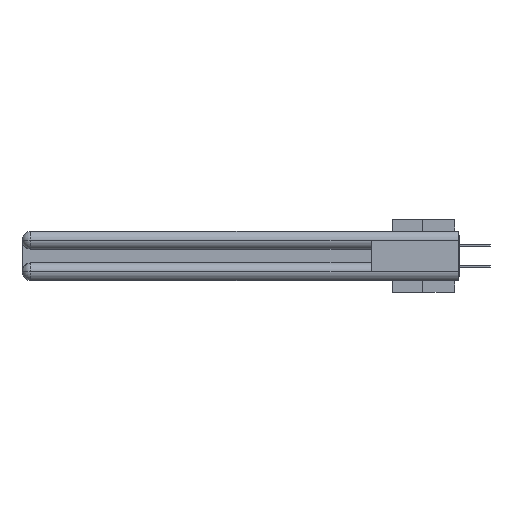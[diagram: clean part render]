
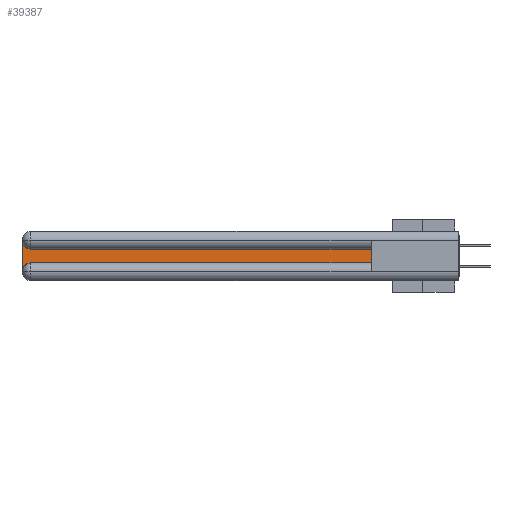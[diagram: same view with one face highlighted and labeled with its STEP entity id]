
A CAD part, left-side view. The second image highlights one B-rep face of the part: STEP entity #39387.
In plain terms, the highlighted planar face has unit normal (-1, 0, 0).
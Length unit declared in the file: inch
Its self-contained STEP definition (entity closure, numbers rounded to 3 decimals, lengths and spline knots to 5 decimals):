
#1821 = LINE ( 'NONE', #38456, #41019 ) ;
#2077 = VERTEX_POINT ( 'NONE', #18280 ) ;
#2661 = VECTOR ( 'NONE', #31508, 39.37008 ) ;
#4078 = LINE ( 'NONE', #7521, #40388 ) ;
#5227 = AXIS2_PLACEMENT_3D ( 'NONE', #21280, #36305, #42930 ) ;
#5736 = CIRCLE ( 'NONE', #5227, 0.06 ) ;
#5887 = CARTESIAN_POINT ( 'NONE',  ( 0.075, 3., -0.2775 ) ) ;
#7521 = CARTESIAN_POINT ( 'NONE',  ( 0.075, 0.6, -0.1225 ) ) ;
#7778 = LINE ( 'NONE', #32529, #10006 ) ;
#8079 = ORIENTED_EDGE ( 'NONE', *, *, #13243, .T. ) ;
#8795 = AXIS2_PLACEMENT_3D ( 'NONE', #41624, #34814, #13100 ) ;
#9459 = PLANE ( 'NONE',  #8795 ) ;
#10006 = VECTOR ( 'NONE', #14460, 39.37008 ) ;
#10050 = VERTEX_POINT ( 'NONE', #34421 ) ;
#11259 = LINE ( 'NONE', #41633, #2661 ) ;
#11621 = CARTESIAN_POINT ( 'NONE',  ( 0.075, 2.94, -0.2175 ) ) ;
#12959 = DIRECTION ( 'NONE',  ( 0., 0., -1. ) ) ;
#13100 = DIRECTION ( 'NONE',  ( 0., 0., -1. ) ) ;
#13243 = EDGE_CURVE ( 'NONE', #30678, #10050, #11259, .T. ) ;
#13375 = FACE_OUTER_BOUND ( 'NONE', #41332, .T. ) ;
#14460 = DIRECTION ( 'NONE',  ( 0., 0., 1. ) ) ;
#14841 = VERTEX_POINT ( 'NONE', #17853 ) ;
#16288 = AXIS2_PLACEMENT_3D ( 'NONE', #17641, #42916, #21264 ) ;
#17641 = CARTESIAN_POINT ( 'NONE',  ( 0.075, 2.94, -0.2775 ) ) ;
#17853 = CARTESIAN_POINT ( 'NONE',  ( 0.075, 2.94, -0.1225 ) ) ;
#18280 = CARTESIAN_POINT ( 'NONE',  ( 0.075, 0.6, -0.1225 ) ) ;
#18743 = CIRCLE ( 'NONE', #16288, 0.06 ) ;
#20013 = ORIENTED_EDGE ( 'NONE', *, *, #34995, .T. ) ;
#21264 = DIRECTION ( 'NONE',  ( 0., 0., -1. ) ) ;
#21280 = CARTESIAN_POINT ( 'NONE',  ( 0.075, 2.94, -0.0625 ) ) ;
#22581 = ORIENTED_EDGE ( 'NONE', *, *, #24065, .T. ) ;
#23924 = VERTEX_POINT ( 'NONE', #5887 ) ;
#24065 = EDGE_CURVE ( 'NONE', #10050, #2077, #7778, .T. ) ;
#24302 = CARTESIAN_POINT ( 'NONE',  ( 0.075, 3., -0.0625 ) ) ;
#25035 = ORIENTED_EDGE ( 'NONE', *, *, #44098, .T. ) ;
#25406 = VERTEX_POINT ( 'NONE', #24302 ) ;
#30678 = VERTEX_POINT ( 'NONE', #11621 ) ;
#31508 = DIRECTION ( 'NONE',  ( 0., -1., 0. ) ) ;
#32529 = CARTESIAN_POINT ( 'NONE',  ( 0.075, 0.6, -0.2175 ) ) ;
#33034 = DIRECTION ( 'NONE',  ( 0., 1., 0. ) ) ;
#34421 = CARTESIAN_POINT ( 'NONE',  ( 0.075, 0.6, -0.2175 ) ) ;
#34814 = DIRECTION ( 'NONE',  ( 1., 0., 0. ) ) ;
#34995 = EDGE_CURVE ( 'NONE', #25406, #23924, #1821, .T. ) ;
#36305 = DIRECTION ( 'NONE',  ( 1., 0., 0. ) ) ;
#38456 = CARTESIAN_POINT ( 'NONE',  ( 0.075, 3., -0.2175 ) ) ;
#39387 = ADVANCED_FACE ( 'NONE', ( #13375 ), #9459, .F. ) ;
#40388 = VECTOR ( 'NONE', #33034, 39.37008 ) ;
#40909 = ORIENTED_EDGE ( 'NONE', *, *, #41760, .T. ) ;
#41019 = VECTOR ( 'NONE', #12959, 39.37008 ) ;
#41332 = EDGE_LOOP ( 'NONE', ( #40909, #41495, #20013, #25035, #8079, #22581 ) ) ;
#41495 = ORIENTED_EDGE ( 'NONE', *, *, #42522, .T. ) ;
#41624 = CARTESIAN_POINT ( 'NONE',  ( 0.075, 3., -0.1225 ) ) ;
#41633 = CARTESIAN_POINT ( 'NONE',  ( 0.075, 0.6, -0.2175 ) ) ;
#41760 = EDGE_CURVE ( 'NONE', #2077, #14841, #4078, .T. ) ;
#42522 = EDGE_CURVE ( 'NONE', #14841, #25406, #5736, .T. ) ;
#42916 = DIRECTION ( 'NONE',  ( 1., 0., 0. ) ) ;
#42930 = DIRECTION ( 'NONE',  ( 0., 0., -1. ) ) ;
#44098 = EDGE_CURVE ( 'NONE', #23924, #30678, #18743, .T. ) ;
